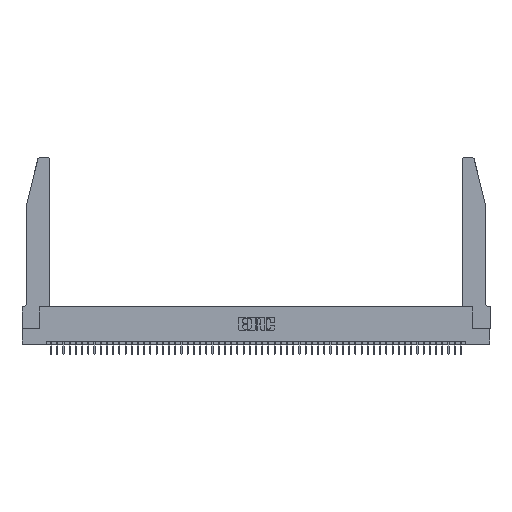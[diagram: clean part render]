
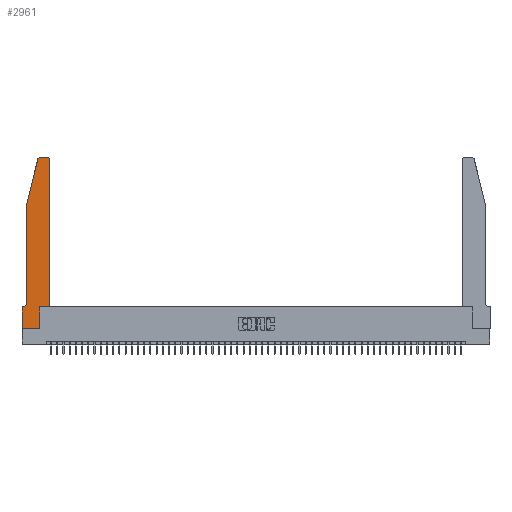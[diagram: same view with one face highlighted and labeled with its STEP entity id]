
A CAD part, top view. The second image highlights one B-rep face of the part: STEP entity #2961.
In plain terms, the highlighted planar face has unit normal (0, 0, 1).
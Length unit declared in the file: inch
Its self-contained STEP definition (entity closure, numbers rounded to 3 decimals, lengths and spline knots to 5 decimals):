
#566 = ORIENTED_EDGE ( 'NONE', *, *, #39678, .T. ) ;
#1228 = LINE ( 'NONE', #22986, #2594 ) ;
#1450 = CIRCLE ( 'NONE', #14238, 0.03 ) ;
#2474 = DIRECTION ( 'NONE',  ( -1., 0., 0. ) ) ;
#2559 = ORIENTED_EDGE ( 'NONE', *, *, #20582, .T. ) ;
#2594 = VECTOR ( 'NONE', #6150, 39.37008 ) ;
#2961 = ADVANCED_FACE ( 'NONE', ( #32304 ), #8040, .T. ) ;
#3092 = LINE ( 'NONE', #24059, #46245 ) ;
#4070 = CARTESIAN_POINT ( 'NONE',  ( 0.2865, 0.35, 0.37 ) ) ;
#5301 = CIRCLE ( 'NONE', #13753, 0.03 ) ;
#5409 = EDGE_CURVE ( 'NONE', #7838, #32629, #3092, .T. ) ;
#6150 = DIRECTION ( 'NONE',  ( 1., 0., 0. ) ) ;
#6837 = EDGE_CURVE ( 'NONE', #30292, #52042, #37776, .T. ) ;
#7838 = VERTEX_POINT ( 'NONE', #20432 ) ;
#8040 = PLANE ( 'NONE',  #18032 ) ;
#9436 = VERTEX_POINT ( 'NONE', #27251 ) ;
#9887 = CARTESIAN_POINT ( 'NONE',  ( 0.0755, 2., 0.37 ) ) ;
#10128 = EDGE_CURVE ( 'NONE', #29692, #7838, #1228, .T. ) ;
#12010 = CARTESIAN_POINT ( 'NONE',  ( 0.4205, 2.72, 0.37 ) ) ;
#12175 = EDGE_CURVE ( 'NONE', #40190, #51942, #27910, .T. ) ;
#13315 = CARTESIAN_POINT ( 'NONE',  ( 0.4205, 2.75, 0.37 ) ) ;
#13753 = AXIS2_PLACEMENT_3D ( 'NONE', #12010, #41196, #16315 ) ;
#14238 = AXIS2_PLACEMENT_3D ( 'NONE', #16326, #45315, #20540 ) ;
#14310 = VECTOR ( 'NONE', #17239, 39.37008 ) ;
#14756 = VECTOR ( 'NONE', #30671, 39.37008 ) ;
#14840 = VECTOR ( 'NONE', #38304, 39.37008 ) ;
#15703 = VECTOR ( 'NONE', #20175, 39.37008 ) ;
#15816 = DIRECTION ( 'NONE',  ( 0., 1., 0. ) ) ;
#15993 = EDGE_LOOP ( 'NONE', ( #35938, #2559, #17400, #24001, #21838, #47064, #16204, #29481, #18319, #19770, #21986, #566 ) ) ;
#16204 = ORIENTED_EDGE ( 'NONE', *, *, #27420, .T. ) ;
#16315 = DIRECTION ( 'NONE',  ( 1., 0., 0. ) ) ;
#16326 = CARTESIAN_POINT ( 'NONE',  ( 0.284, 2.72, 0.37 ) ) ;
#16609 = DIRECTION ( 'NONE',  ( 1., 0., 0. ) ) ;
#17239 = DIRECTION ( 'NONE',  ( 0., -1., 0. ) ) ;
#17390 = CARTESIAN_POINT ( 'NONE',  ( 0.4505, 0.35, 0.37 ) ) ;
#17400 = ORIENTED_EDGE ( 'NONE', *, *, #26672, .T. ) ;
#18032 = AXIS2_PLACEMENT_3D ( 'NONE', #37330, #41473, #16609 ) ;
#18319 = ORIENTED_EDGE ( 'NONE', *, *, #5409, .T. ) ;
#19770 = ORIENTED_EDGE ( 'NONE', *, *, #51013, .T. ) ;
#19862 = CARTESIAN_POINT ( 'NONE',  ( 0.0755, 2., 0.37 ) ) ;
#20175 = DIRECTION ( 'NONE',  ( 0., -1., 0. ) ) ;
#20432 = CARTESIAN_POINT ( 'NONE',  ( 0.2865, 0., 0.37 ) ) ;
#20540 = DIRECTION ( 'NONE',  ( 1., 0., 0. ) ) ;
#20582 = EDGE_CURVE ( 'NONE', #42710, #42658, #1450, .T. ) ;
#20698 = EDGE_CURVE ( 'NONE', #48484, #42710, #39559, .T. ) ;
#21170 = EDGE_CURVE ( 'NONE', #43263, #9436, #27227, .T. ) ;
#21838 = ORIENTED_EDGE ( 'NONE', *, *, #40206, .T. ) ;
#21986 = ORIENTED_EDGE ( 'NONE', *, *, #12175, .T. ) ;
#22986 = CARTESIAN_POINT ( 'NONE',  ( 0., 0., 0.37 ) ) ;
#23431 = CARTESIAN_POINT ( 'NONE',  ( 0.4505, 0.35, 0.37 ) ) ;
#24001 = ORIENTED_EDGE ( 'NONE', *, *, #6837, .T. ) ;
#24059 = CARTESIAN_POINT ( 'NONE',  ( 0.2865, 0.35, 0.37 ) ) ;
#25116 = CARTESIAN_POINT ( 'NONE',  ( 0.0055, 0.35, 0.37 ) ) ;
#25519 = LINE ( 'NONE', #44961, #15703 ) ;
#25983 = LINE ( 'NONE', #17390, #14840 ) ;
#26672 = EDGE_CURVE ( 'NONE', #42658, #30292, #41135, .T. ) ;
#27227 = LINE ( 'NONE', #51131, #14756 ) ;
#27251 = CARTESIAN_POINT ( 'NONE',  ( 0., 0.35, 0.37 ) ) ;
#27309 = DIRECTION ( 'NONE',  ( 0., 1., 0. ) ) ;
#27376 = CARTESIAN_POINT ( 'NONE',  ( 0.4505, 2.72, 0.37 ) ) ;
#27420 = EDGE_CURVE ( 'NONE', #9436, #29692, #25519, .T. ) ;
#27808 = DIRECTION ( 'NONE',  ( 0., 0., -1. ) ) ;
#27910 = LINE ( 'NONE', #47797, #48488 ) ;
#29481 = ORIENTED_EDGE ( 'NONE', *, *, #10128, .T. ) ;
#29692 = VERTEX_POINT ( 'NONE', #39026 ) ;
#30292 = VERTEX_POINT ( 'NONE', #9887 ) ;
#30671 = DIRECTION ( 'NONE',  ( -1., 0., 0. ) ) ;
#32304 = FACE_OUTER_BOUND ( 'NONE', #15993, .T. ) ;
#32347 = AXIS2_PLACEMENT_3D ( 'NONE', #52424, #27808, #2474 ) ;
#32629 = VERTEX_POINT ( 'NONE', #4070 ) ;
#33830 = CARTESIAN_POINT ( 'NONE',  ( 0.0755, 2., 0.37 ) ) ;
#35938 = ORIENTED_EDGE ( 'NONE', *, *, #20698, .T. ) ;
#36400 = CARTESIAN_POINT ( 'NONE',  ( 0.0755, 0.42, 0.37 ) ) ;
#37330 = CARTESIAN_POINT ( 'NONE',  ( 0., 0.35, 0.37 ) ) ;
#37776 = LINE ( 'NONE', #33830, #14310 ) ;
#37960 = DIRECTION ( 'NONE',  ( -1., 0., 0. ) ) ;
#38237 = CARTESIAN_POINT ( 'NONE',  ( 0.25487, 2.72718, 0.37 ) ) ;
#38273 = VECTOR ( 'NONE', #37960, 39.37008 ) ;
#38304 = DIRECTION ( 'NONE',  ( 1., 0., 0. ) ) ;
#39026 = CARTESIAN_POINT ( 'NONE',  ( 0., 0., 0.37 ) ) ;
#39559 = LINE ( 'NONE', #41921, #38273 ) ;
#39678 = EDGE_CURVE ( 'NONE', #51942, #48484, #5301, .T. ) ;
#40190 = VERTEX_POINT ( 'NONE', #23431 ) ;
#40206 = EDGE_CURVE ( 'NONE', #52042, #43263, #54038, .T. ) ;
#41135 = LINE ( 'NONE', #19862, #52022 ) ;
#41196 = DIRECTION ( 'NONE',  ( 0., 0., 1. ) ) ;
#41473 = DIRECTION ( 'NONE',  ( 0., 0., 1. ) ) ;
#41921 = CARTESIAN_POINT ( 'NONE',  ( 0.2605, 2.75, 0.37 ) ) ;
#42528 = CARTESIAN_POINT ( 'NONE',  ( 0.284, 2.75, 0.37 ) ) ;
#42658 = VERTEX_POINT ( 'NONE', #38237 ) ;
#42710 = VERTEX_POINT ( 'NONE', #42528 ) ;
#43263 = VERTEX_POINT ( 'NONE', #25116 ) ;
#44961 = CARTESIAN_POINT ( 'NONE',  ( 0., 0., 0.37 ) ) ;
#45315 = DIRECTION ( 'NONE',  ( 0., 0., 1. ) ) ;
#46245 = VECTOR ( 'NONE', #15816, 39.37008 ) ;
#47064 = ORIENTED_EDGE ( 'NONE', *, *, #21170, .T. ) ;
#47797 = CARTESIAN_POINT ( 'NONE',  ( 0.4505, 0.35, 0.37 ) ) ;
#48484 = VERTEX_POINT ( 'NONE', #13315 ) ;
#48488 = VECTOR ( 'NONE', #27309, 39.37008 ) ;
#48746 = DIRECTION ( 'NONE',  ( -0.239, -0.971, 0. ) ) ;
#51013 = EDGE_CURVE ( 'NONE', #32629, #40190, #25983, .T. ) ;
#51131 = CARTESIAN_POINT ( 'NONE',  ( 0.0755, 0.35, 0.37 ) ) ;
#51942 = VERTEX_POINT ( 'NONE', #27376 ) ;
#52022 = VECTOR ( 'NONE', #48746, 39.37008 ) ;
#52042 = VERTEX_POINT ( 'NONE', #36400 ) ;
#52424 = CARTESIAN_POINT ( 'NONE',  ( 0.0055, 0.42, 0.37 ) ) ;
#54038 = CIRCLE ( 'NONE', #32347, 0.07 ) ;
